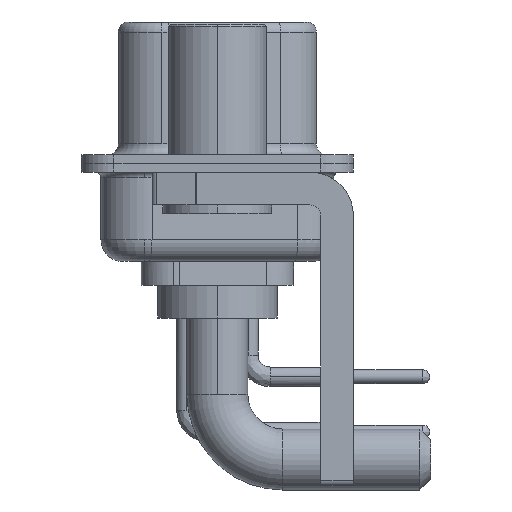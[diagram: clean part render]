
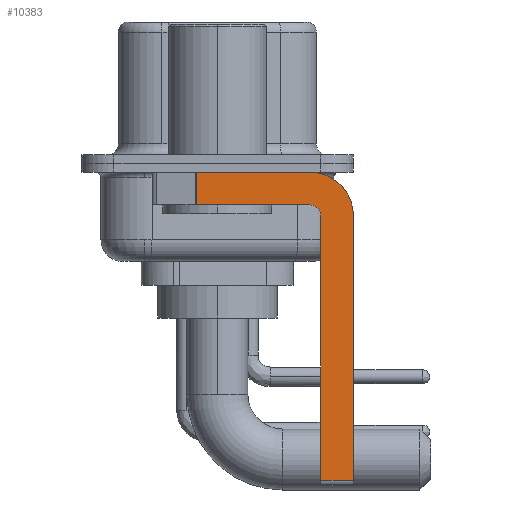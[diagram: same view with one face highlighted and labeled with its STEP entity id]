
A CAD part, left-side view. The second image highlights one B-rep face of the part: STEP entity #10383.
In plain terms, the highlighted planar face has unit normal (-1, 0, 0).
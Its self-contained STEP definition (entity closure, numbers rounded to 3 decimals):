
#72 = DIRECTION ( 'NONE',  ( 0., 0., -1. ) ) ;
#708 = DIRECTION ( 'NONE',  ( -1., 0., 0. ) ) ;
#726 = CARTESIAN_POINT ( 'NONE',  ( -2.9, 3., -0.4 ) ) ;
#740 = CARTESIAN_POINT ( 'NONE',  ( -2.9, -4.75, -14.55 ) ) ;
#959 = CARTESIAN_POINT ( 'NONE',  ( -2.9, 0.978, -0.4 ) ) ;
#1135 = LINE ( 'NONE', #14530, #20984 ) ;
#1737 = CARTESIAN_POINT ( 'NONE',  ( -2.9, 0.978, -1.9 ) ) ;
#2792 = DIRECTION ( 'NONE',  ( 0., 0., -1. ) ) ;
#3016 = EDGE_CURVE ( 'NONE', #22324, #21453, #20145, .T. ) ;
#3323 = DIRECTION ( 'NONE',  ( 0., 0., -1. ) ) ;
#3718 = AXIS2_PLACEMENT_3D ( 'NONE', #9392, #708, #22161 ) ;
#3843 = DIRECTION ( 'NONE',  ( 0., 0., -1. ) ) ;
#3848 = DIRECTION ( 'NONE',  ( 0., 0., 1. ) ) ;
#3883 = DIRECTION ( 'NONE',  ( 0., 1., 0. ) ) ;
#4390 = LINE ( 'NONE', #726, #4392 ) ;
#4392 = VECTOR ( 'NONE', #13296, 1000. ) ;
#4773 = EDGE_CURVE ( 'NONE', #20925, #21453, #19759, .T. ) ;
#6195 = ORIENTED_EDGE ( 'NONE', *, *, #4773, .T. ) ;
#6348 = CIRCLE ( 'NONE', #3718, 0.5 ) ;
#6522 = VERTEX_POINT ( 'NONE', #11244 ) ;
#7981 = ORIENTED_EDGE ( 'NONE', *, *, #15668, .T. ) ;
#8017 = CARTESIAN_POINT ( 'NONE',  ( -2.9, -4.25, -0.4 ) ) ;
#8231 = ORIENTED_EDGE ( 'NONE', *, *, #19002, .F. ) ;
#8352 = VECTOR ( 'NONE', #3883, 1000. ) ;
#8435 = ORIENTED_EDGE ( 'NONE', *, *, #19644, .F. ) ;
#8502 = EDGE_CURVE ( 'NONE', #6522, #18621, #1135, .T. ) ;
#8862 = CARTESIAN_POINT ( 'NONE',  ( -2.9, -4.25, -1.9 ) ) ;
#9392 = CARTESIAN_POINT ( 'NONE',  ( -2.9, -4.25, -2.4 ) ) ;
#9472 = VECTOR ( 'NONE', #15964, 1000. ) ;
#9787 = CIRCLE ( 'NONE', #21900, 2. ) ;
#9885 = CARTESIAN_POINT ( 'NONE',  ( -2.9, -4.25, -2.4 ) ) ;
#10065 = CARTESIAN_POINT ( 'NONE',  ( -2.9, 0.978, -1.9 ) ) ;
#10383 = ADVANCED_FACE ( 'NONE', ( #15723 ), #22597, .F. ) ;
#10799 = EDGE_LOOP ( 'NONE', ( #8435, #6195, #15567, #23015, #8231, #7981, #17225, #14032 ) ) ;
#10827 = AXIS2_PLACEMENT_3D ( 'NONE', #19039, #15602, #2792 ) ;
#11244 = CARTESIAN_POINT ( 'NONE',  ( -2.9, -6.25, -2.4 ) ) ;
#11462 = CARTESIAN_POINT ( 'NONE',  ( -2.9, -4.25, -1.9 ) ) ;
#12295 = CARTESIAN_POINT ( 'NONE',  ( -2.9, -4.75, -2.4 ) ) ;
#13296 = DIRECTION ( 'NONE',  ( 0., -1., 0. ) ) ;
#13911 = VERTEX_POINT ( 'NONE', #8017 ) ;
#14032 = ORIENTED_EDGE ( 'NONE', *, *, #22136, .F. ) ;
#14163 = EDGE_CURVE ( 'NONE', #18271, #22324, #6348, .T. ) ;
#14530 = CARTESIAN_POINT ( 'NONE',  ( -2.9, -6.25, -2.4 ) ) ;
#15329 = DIRECTION ( 'NONE',  ( 1., 0., 0. ) ) ;
#15567 = ORIENTED_EDGE ( 'NONE', *, *, #3016, .F. ) ;
#15602 = DIRECTION ( 'NONE',  ( 1., 0., 0. ) ) ;
#15668 = EDGE_CURVE ( 'NONE', #22855, #18621, #21288, .T. ) ;
#15723 = FACE_OUTER_BOUND ( 'NONE', #10799, .T. ) ;
#15964 = DIRECTION ( 'NONE',  ( 0., -1., 0. ) ) ;
#17225 = ORIENTED_EDGE ( 'NONE', *, *, #8502, .F. ) ;
#18271 = VERTEX_POINT ( 'NONE', #12295 ) ;
#18318 = CARTESIAN_POINT ( 'NONE',  ( -2.9, -4.75, -14.8 ) ) ;
#18621 = VERTEX_POINT ( 'NONE', #18925 ) ;
#18925 = CARTESIAN_POINT ( 'NONE',  ( -2.9, -6.25, -14.55 ) ) ;
#19002 = EDGE_CURVE ( 'NONE', #22855, #18271, #22211, .T. ) ;
#19039 = CARTESIAN_POINT ( 'NONE',  ( -2.9, -4.25, -2.4 ) ) ;
#19501 = CARTESIAN_POINT ( 'NONE',  ( -2.9, -4.25, -14.55 ) ) ;
#19644 = EDGE_CURVE ( 'NONE', #20925, #13911, #4390, .T. ) ;
#19759 = LINE ( 'NONE', #1737, #22507 ) ;
#20145 = LINE ( 'NONE', #11462, #8352 ) ;
#20925 = VERTEX_POINT ( 'NONE', #959 ) ;
#20984 = VECTOR ( 'NONE', #3843, 1000. ) ;
#21288 = LINE ( 'NONE', #19501, #9472 ) ;
#21453 = VERTEX_POINT ( 'NONE', #10065 ) ;
#21900 = AXIS2_PLACEMENT_3D ( 'NONE', #9885, #15329, #3323 ) ;
#22136 = EDGE_CURVE ( 'NONE', #13911, #6522, #9787, .T. ) ;
#22161 = DIRECTION ( 'NONE',  ( 0., 0., 1. ) ) ;
#22211 = LINE ( 'NONE', #18318, #22560 ) ;
#22324 = VERTEX_POINT ( 'NONE', #8862 ) ;
#22507 = VECTOR ( 'NONE', #72, 1000. ) ;
#22560 = VECTOR ( 'NONE', #3848, 1000. ) ;
#22597 = PLANE ( 'NONE',  #10827 ) ;
#22855 = VERTEX_POINT ( 'NONE', #740 ) ;
#23015 = ORIENTED_EDGE ( 'NONE', *, *, #14163, .F. ) ;
